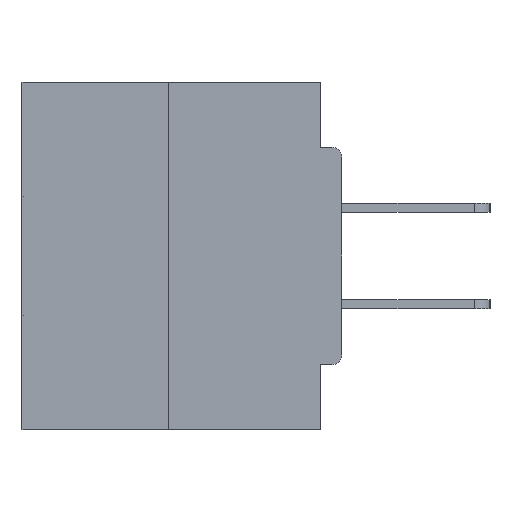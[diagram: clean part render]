
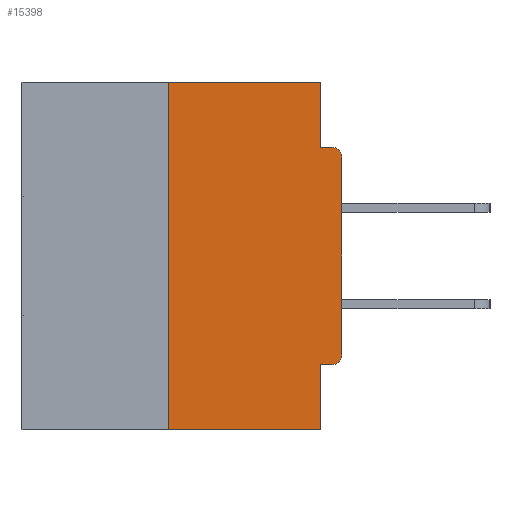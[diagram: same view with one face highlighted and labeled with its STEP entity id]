
A CAD part, left-side view. The second image highlights one B-rep face of the part: STEP entity #15398.
In plain terms, the highlighted planar face has unit normal (-1, 0, 0).
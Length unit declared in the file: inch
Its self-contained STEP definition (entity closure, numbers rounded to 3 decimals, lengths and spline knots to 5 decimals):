
#1053 = EDGE_LOOP ( 'NONE', ( #17182, #4052, #24437, #4851, #25094, #8780, #13736, #15203, #12431, #4254 ) ) ;
#1438 = EDGE_CURVE ( 'NONE', #12293, #2528, #24983, .T. ) ;
#2088 = VECTOR ( 'NONE', #6313, 39.37008 ) ;
#2151 = EDGE_CURVE ( 'NONE', #14116, #33258, #35367, .T. ) ;
#2528 = VERTEX_POINT ( 'NONE', #23229 ) ;
#3346 = EDGE_CURVE ( 'NONE', #2528, #14116, #6638, .T. ) ;
#3773 = CARTESIAN_POINT ( 'NONE',  ( 0., 0.031, -0.5 ) ) ;
#4052 = ORIENTED_EDGE ( 'NONE', *, *, #34397, .F. ) ;
#4254 = ORIENTED_EDGE ( 'NONE', *, *, #15208, .F. ) ;
#4851 = ORIENTED_EDGE ( 'NONE', *, *, #37491, .F. ) ;
#6313 = DIRECTION ( 'NONE',  ( 0., 0., -1. ) ) ;
#6549 = CARTESIAN_POINT ( 'NONE',  ( 0., 0.031, -0.5 ) ) ;
#6638 = LINE ( 'NONE', #24433, #9483 ) ;
#6802 = CARTESIAN_POINT ( 'NONE',  ( 0., 0.031, 0. ) ) ;
#7567 = DIRECTION ( 'NONE',  ( 0., 0., -1. ) ) ;
#8516 = VECTOR ( 'NONE', #14362, 39.37008 ) ;
#8780 = ORIENTED_EDGE ( 'NONE', *, *, #1438, .T. ) ;
#9483 = VECTOR ( 'NONE', #31795, 39.37008 ) ;
#9589 = CARTESIAN_POINT ( 'NONE',  ( 0., 0.031, -0.4065 ) ) ;
#10880 = CARTESIAN_POINT ( 'NONE',  ( 0., 0.46, -0.5 ) ) ;
#10909 = VECTOR ( 'NONE', #36162, 39.37008 ) ;
#11299 = VERTEX_POINT ( 'NONE', #13025 ) ;
#11826 = VERTEX_POINT ( 'NONE', #35197 ) ;
#12212 = CARTESIAN_POINT ( 'NONE',  ( 0., 0.031, -0.0935 ) ) ;
#12293 = VERTEX_POINT ( 'NONE', #34129 ) ;
#12431 = ORIENTED_EDGE ( 'NONE', *, *, #14163, .F. ) ;
#13025 = CARTESIAN_POINT ( 'NONE',  ( 0., 0.25, -0.5 ) ) ;
#13225 = DIRECTION ( 'NONE',  ( 0., 0., -1. ) ) ;
#13736 = ORIENTED_EDGE ( 'NONE', *, *, #3346, .T. ) ;
#13758 = DIRECTION ( 'NONE',  ( 1., 0., 0. ) ) ;
#13785 = LINE ( 'NONE', #10880, #18487 ) ;
#13787 = LINE ( 'NONE', #6802, #2088 ) ;
#14116 = VERTEX_POINT ( 'NONE', #21883 ) ;
#14163 = EDGE_CURVE ( 'NONE', #29688, #33258, #38274, .T. ) ;
#14362 = DIRECTION ( 'NONE',  ( 0., 1., 0. ) ) ;
#14609 = LINE ( 'NONE', #17496, #8516 ) ;
#14869 = DIRECTION ( 'NONE',  ( 0., -1., 0. ) ) ;
#15180 = AXIS2_PLACEMENT_3D ( 'NONE', #30732, #33651, #13225 ) ;
#15203 = ORIENTED_EDGE ( 'NONE', *, *, #2151, .T. ) ;
#15208 = EDGE_CURVE ( 'NONE', #29748, #29688, #13787, .T. ) ;
#15398 = ADVANCED_FACE ( 'NONE', ( #32032 ), #35502, .F. ) ;
#17182 = ORIENTED_EDGE ( 'NONE', *, *, #36604, .F. ) ;
#17496 = CARTESIAN_POINT ( 'NONE',  ( 0., 0., -0.4065 ) ) ;
#18487 = VECTOR ( 'NONE', #31786, 39.37008 ) ;
#18556 = VECTOR ( 'NONE', #19130, 39.37008 ) ;
#18922 = DIRECTION ( 'NONE',  ( 0., 0., -1. ) ) ;
#19130 = DIRECTION ( 'NONE',  ( 0., -1., 0. ) ) ;
#19712 = CARTESIAN_POINT ( 'NONE',  ( 0., 0.46, 0. ) ) ;
#19764 = CARTESIAN_POINT ( 'NONE',  ( 0., 0.46, 0. ) ) ;
#21798 = DIRECTION ( 'NONE',  ( -1., 0., 0. ) ) ;
#21883 = CARTESIAN_POINT ( 'NONE',  ( 0., 0., -0.1085 ) ) ;
#22209 = VECTOR ( 'NONE', #14869, 39.37008 ) ;
#22582 = LINE ( 'NONE', #6549, #10909 ) ;
#22917 = CARTESIAN_POINT ( 'NONE',  ( 0., 0.25, 0. ) ) ;
#23229 = CARTESIAN_POINT ( 'NONE',  ( 0., 0., -0.3915 ) ) ;
#24433 = CARTESIAN_POINT ( 'NONE',  ( 0., 0., 0. ) ) ;
#24437 = ORIENTED_EDGE ( 'NONE', *, *, #24720, .T. ) ;
#24720 = EDGE_CURVE ( 'NONE', #11299, #26819, #13785, .T. ) ;
#24983 = CIRCLE ( 'NONE', #15180, 0.015 ) ;
#25094 = ORIENTED_EDGE ( 'NONE', *, *, #37967, .F. ) ;
#26166 = VECTOR ( 'NONE', #26197, 39.37008 ) ;
#26197 = DIRECTION ( 'NONE',  ( 0., 0., 1. ) ) ;
#26819 = VERTEX_POINT ( 'NONE', #3773 ) ;
#28141 = AXIS2_PLACEMENT_3D ( 'NONE', #19764, #13758, #7567 ) ;
#29561 = CARTESIAN_POINT ( 'NONE',  ( 0., 0.015, -0.0935 ) ) ;
#29688 = VERTEX_POINT ( 'NONE', #12212 ) ;
#29748 = VERTEX_POINT ( 'NONE', #34520 ) ;
#30732 = CARTESIAN_POINT ( 'NONE',  ( 0., 0.015, -0.3915 ) ) ;
#30866 = VERTEX_POINT ( 'NONE', #9589 ) ;
#31786 = DIRECTION ( 'NONE',  ( 0., -1., 0. ) ) ;
#31795 = DIRECTION ( 'NONE',  ( 0., 0., 1. ) ) ;
#32032 = FACE_OUTER_BOUND ( 'NONE', #1053, .T. ) ;
#33017 = AXIS2_PLACEMENT_3D ( 'NONE', #37234, #21798, #18922 ) ;
#33258 = VERTEX_POINT ( 'NONE', #29561 ) ;
#33651 = DIRECTION ( 'NONE',  ( -1., 0., 0. ) ) ;
#34116 = LINE ( 'NONE', #22917, #26166 ) ;
#34129 = CARTESIAN_POINT ( 'NONE',  ( 0., 0.015, -0.4065 ) ) ;
#34397 = EDGE_CURVE ( 'NONE', #11299, #11826, #34116, .T. ) ;
#34520 = CARTESIAN_POINT ( 'NONE',  ( 0., 0.031, 0. ) ) ;
#35197 = CARTESIAN_POINT ( 'NONE',  ( 0., 0.25, 0. ) ) ;
#35354 = LINE ( 'NONE', #19712, #22209 ) ;
#35367 = CIRCLE ( 'NONE', #33017, 0.015 ) ;
#35502 = PLANE ( 'NONE',  #28141 ) ;
#36162 = DIRECTION ( 'NONE',  ( 0., 0., -1. ) ) ;
#36604 = EDGE_CURVE ( 'NONE', #11826, #29748, #35354, .T. ) ;
#37189 = CARTESIAN_POINT ( 'NONE',  ( 0., 0., -0.0935 ) ) ;
#37234 = CARTESIAN_POINT ( 'NONE',  ( 0., 0.015, -0.1085 ) ) ;
#37491 = EDGE_CURVE ( 'NONE', #30866, #26819, #22582, .T. ) ;
#37967 = EDGE_CURVE ( 'NONE', #12293, #30866, #14609, .T. ) ;
#38274 = LINE ( 'NONE', #37189, #18556 ) ;
